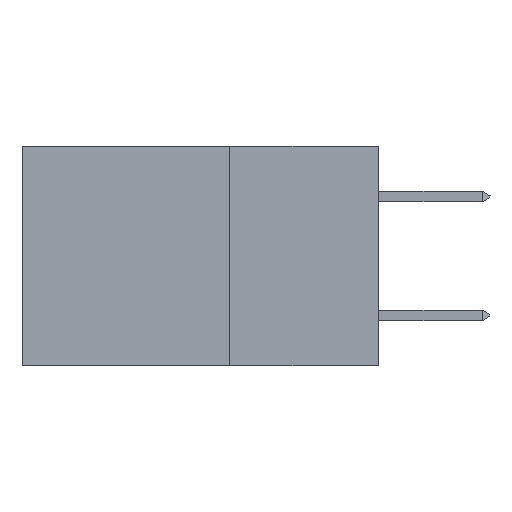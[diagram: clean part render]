
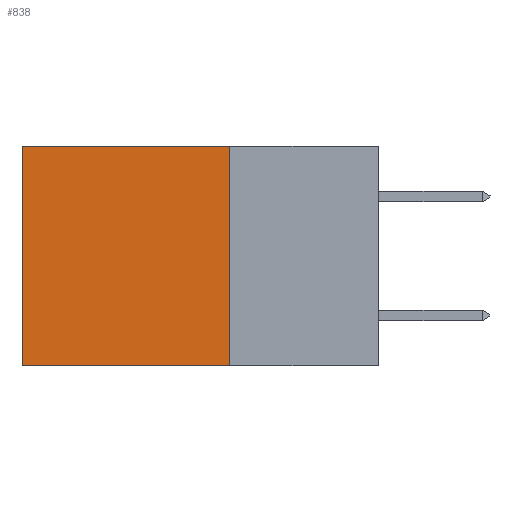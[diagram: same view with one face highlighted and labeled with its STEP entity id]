
A CAD part, left-side view. The second image highlights one B-rep face of the part: STEP entity #838.
In plain terms, the highlighted planar face has unit normal (-1, 0, 0).
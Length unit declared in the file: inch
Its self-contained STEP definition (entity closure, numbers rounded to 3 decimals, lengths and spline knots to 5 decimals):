
#99 = LINE ( 'NONE', #322, #3153 ) ;
#176 = CARTESIAN_POINT ( 'NONE',  ( 0.2615, 0.6, -0.37 ) ) ;
#322 = CARTESIAN_POINT ( 'NONE',  ( 0.2615, 0.25, -0.37 ) ) ;
#616 = DIRECTION ( 'NONE',  ( 1., 0., 0. ) ) ;
#674 = ORIENTED_EDGE ( 'NONE', *, *, #9576, .T. ) ;
#838 = ADVANCED_FACE ( 'NONE', ( #1491 ), #1732, .F. ) ;
#1199 = CARTESIAN_POINT ( 'NONE',  ( 0.2615, 0.25, 0. ) ) ;
#1253 = LINE ( 'NONE', #7866, #3207 ) ;
#1491 = FACE_OUTER_BOUND ( 'NONE', #8532, .T. ) ;
#1732 = PLANE ( 'NONE',  #8959 ) ;
#2730 = CARTESIAN_POINT ( 'NONE',  ( 0.2615, 0.6, 0. ) ) ;
#3142 = VECTOR ( 'NONE', #5009, 39.37008 ) ;
#3147 = LINE ( 'NONE', #1199, #3142 ) ;
#3153 = VECTOR ( 'NONE', #5207, 39.37008 ) ;
#3207 = VECTOR ( 'NONE', #4005, 39.37008 ) ;
#3416 = LINE ( 'NONE', #7204, #8664 ) ;
#3998 = EDGE_CURVE ( 'NONE', #4195, #9161, #1253, .T. ) ;
#4005 = DIRECTION ( 'NONE',  ( 0., 0., -1. ) ) ;
#4089 = CARTESIAN_POINT ( 'NONE',  ( 0.2615, 0.25, -0.37 ) ) ;
#4195 = VERTEX_POINT ( 'NONE', #10352 ) ;
#4368 = CARTESIAN_POINT ( 'NONE',  ( 0.2615, 0.25, -0.37 ) ) ;
#5009 = DIRECTION ( 'NONE',  ( 0., 1., 0. ) ) ;
#5143 = ORIENTED_EDGE ( 'NONE', *, *, #12160, .F. ) ;
#5207 = DIRECTION ( 'NONE',  ( 0., 1., 0. ) ) ;
#7204 = CARTESIAN_POINT ( 'NONE',  ( 0.2615, 0.6, -0.37 ) ) ;
#7866 = CARTESIAN_POINT ( 'NONE',  ( 0.2615, 0.25, -0.37 ) ) ;
#8158 = EDGE_CURVE ( 'NONE', #10138, #11748, #3416, .T. ) ;
#8532 = EDGE_LOOP ( 'NONE', ( #9155, #5143, #9486, #674 ) ) ;
#8664 = VECTOR ( 'NONE', #8998, 39.37008 ) ;
#8959 = AXIS2_PLACEMENT_3D ( 'NONE', #4368, #616, #10907 ) ;
#8998 = DIRECTION ( 'NONE',  ( 0., 0., -1. ) ) ;
#9155 = ORIENTED_EDGE ( 'NONE', *, *, #8158, .T. ) ;
#9161 = VERTEX_POINT ( 'NONE', #4089 ) ;
#9486 = ORIENTED_EDGE ( 'NONE', *, *, #3998, .F. ) ;
#9576 = EDGE_CURVE ( 'NONE', #4195, #10138, #3147, .T. ) ;
#10138 = VERTEX_POINT ( 'NONE', #2730 ) ;
#10352 = CARTESIAN_POINT ( 'NONE',  ( 0.2615, 0.25, 0. ) ) ;
#10907 = DIRECTION ( 'NONE',  ( 0., 0., -1. ) ) ;
#11748 = VERTEX_POINT ( 'NONE', #176 ) ;
#12160 = EDGE_CURVE ( 'NONE', #9161, #11748, #99, .T. ) ;
